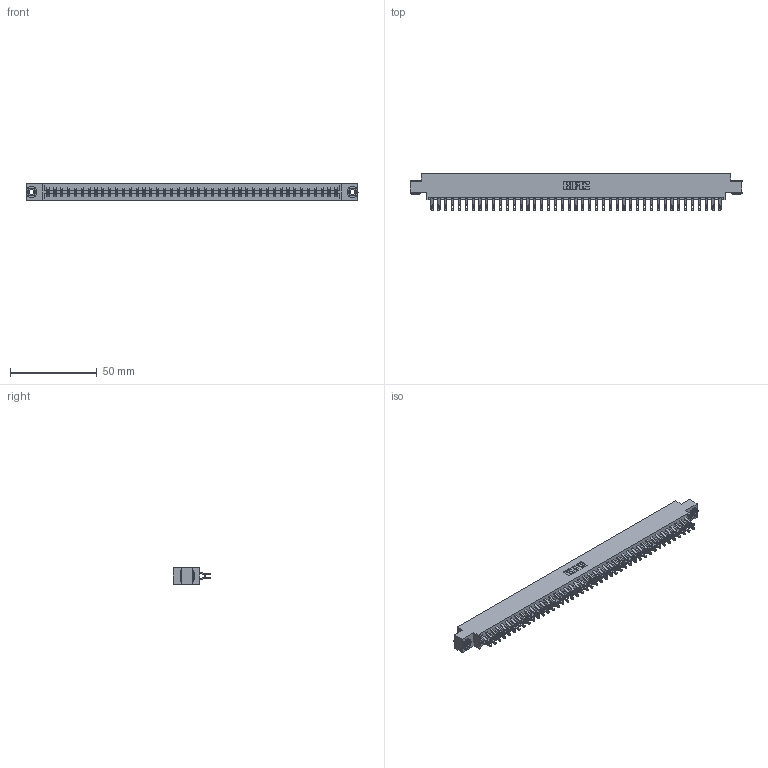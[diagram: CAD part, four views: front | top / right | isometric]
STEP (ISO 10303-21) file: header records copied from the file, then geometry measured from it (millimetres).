
FILE_DESCRIPTION (( 'STEP AP203' ), '1' );
FILE_NAME ('333-086-555-803.STEP', '2018-08-05T06:39:51', ( '' ), ( '' ), 'SwSTEP 2.0', 'SolidWorks 2016', '' );
FILE_SCHEMA (( 'CONFIG_CONTROL_DESIGN' ));
Length unit declared in the file: inch
Products named in the file (4): 345-292-001_555 Tail; 345-250-002_345-250-002-102; 333-086-555-803; 333 Part_Offset - .156 Dia - TH
Assembly tree (89 placements, depth 2):
  333-086-555-803
    333 Part_Offset - .156 Dia - TH
    345-292-001_555 Tail  x86
    345-250-002_345-250-002-102  x2
Bounding box: 191.92 x 21.47 x 9.4 mm (x, y, z)
Volume: 19644.6 mm3; surface area: 24610.1 mm2
Topology: 89 solids, 89 shells, 5144 faces, 16137 edges, 10754 vertices
Faces by surface type: plane 3008, cylinder 2128, cone 8
Entity records: 28642 total; most frequent: CARTESIAN_POINT 4759, ORIENTED_EDGE 4658, DIRECTION 4067, EDGE_CURVE 2329, VECTOR 2157, LINE 2157, VERTEX_POINT 1550, AXIS2_PLACEMENT_3D 955
